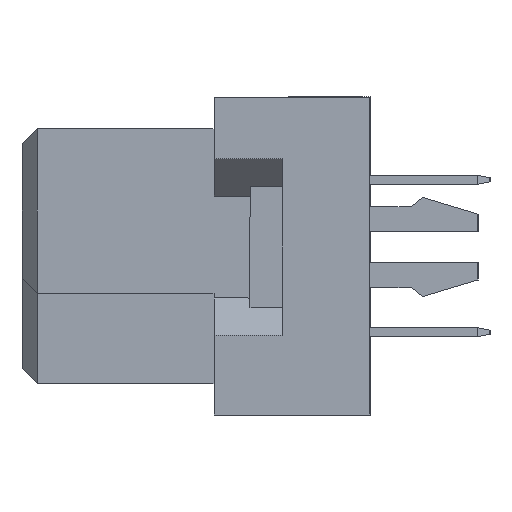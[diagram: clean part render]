
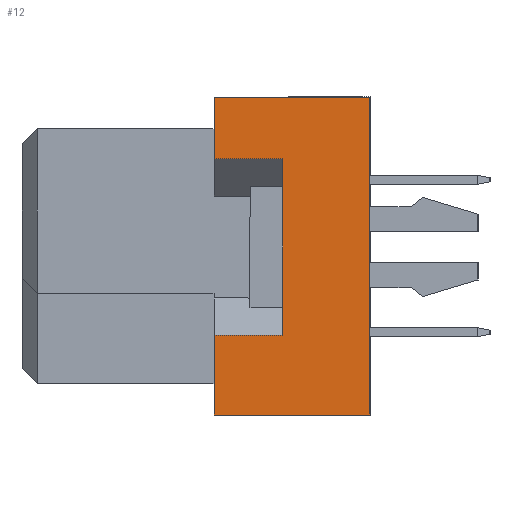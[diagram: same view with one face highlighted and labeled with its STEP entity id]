
A CAD part, left-side view. The second image highlights one B-rep face of the part: STEP entity #12.
In plain terms, the highlighted planar face has unit normal (-1, 0, 0).
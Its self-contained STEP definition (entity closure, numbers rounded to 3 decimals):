
#12 = ADVANCED_FACE ( 'NONE', ( #2517 ), #5895, .T. ) ;
#222 = EDGE_CURVE ( 'NONE', #2448, #16559, #4938, .T. ) ;
#498 = DIRECTION ( 'NONE',  ( 0., 0., 1. ) ) ;
#691 = EDGE_CURVE ( 'NONE', #2448, #20580, #8962, .T. ) ;
#697 = DIRECTION ( 'NONE',  ( 0., 0., 1. ) ) ;
#1095 = CARTESIAN_POINT ( 'NONE',  ( -27.5, -8.7, 3.25 ) ) ;
#1193 = DIRECTION ( 'NONE',  ( 0., 1., 0. ) ) ;
#1994 = VERTEX_POINT ( 'NONE', #15630 ) ;
#2054 = VECTOR ( 'NONE', #9783, 1000. ) ;
#2367 = VECTOR ( 'NONE', #697, 1000. ) ;
#2448 = VERTEX_POINT ( 'NONE', #15815 ) ;
#2517 = FACE_OUTER_BOUND ( 'NONE', #18444, .T. ) ;
#2866 = VERTEX_POINT ( 'NONE', #7513 ) ;
#3087 = VECTOR ( 'NONE', #9484, 1000. ) ;
#3811 = VECTOR ( 'NONE', #498, 1000. ) ;
#3842 = CARTESIAN_POINT ( 'NONE',  ( -27.5, -11.6, -5.3 ) ) ;
#3934 = ORIENTED_EDGE ( 'NONE', *, *, #18700, .T. ) ;
#4005 = AXIS2_PLACEMENT_3D ( 'NONE', #10819, #9157, #9797 ) ;
#4315 = ORIENTED_EDGE ( 'NONE', *, *, #8371, .F. ) ;
#4316 = VECTOR ( 'NONE', #1193, 1000. ) ;
#4778 = LINE ( 'NONE', #1095, #4316 ) ;
#4833 = CARTESIAN_POINT ( 'NONE',  ( -27.5, -11.6, 5.3 ) ) ;
#4938 = LINE ( 'NONE', #4833, #7492 ) ;
#4966 = CARTESIAN_POINT ( 'NONE',  ( -27.5, -11.6, 5.3 ) ) ;
#5068 = CARTESIAN_POINT ( 'NONE',  ( -27.5, -8.7, -2.65 ) ) ;
#5236 = CARTESIAN_POINT ( 'NONE',  ( -27.5, -11.6, 5.3 ) ) ;
#5796 = DIRECTION ( 'NONE',  ( 0., 1., 0. ) ) ;
#5895 = PLANE ( 'NONE',  #4005 ) ;
#6091 = VERTEX_POINT ( 'NONE', #11213 ) ;
#6583 = DIRECTION ( 'NONE',  ( 0., 0., 1. ) ) ;
#6626 = ORIENTED_EDGE ( 'NONE', *, *, #222, .T. ) ;
#7226 = EDGE_CURVE ( 'NONE', #2866, #18574, #7423, .T. ) ;
#7423 = LINE ( 'NONE', #11024, #3087 ) ;
#7492 = VECTOR ( 'NONE', #6583, 1000. ) ;
#7513 = CARTESIAN_POINT ( 'NONE',  ( -27.5, -8.7, -2.65 ) ) ;
#7664 = CARTESIAN_POINT ( 'NONE',  ( -27.5, -6.4, -5.3 ) ) ;
#7937 = ORIENTED_EDGE ( 'NONE', *, *, #13612, .F. ) ;
#8371 = EDGE_CURVE ( 'NONE', #2866, #1994, #13483, .T. ) ;
#8962 = LINE ( 'NONE', #3842, #12075 ) ;
#9157 = DIRECTION ( 'NONE',  ( -1., 0., 0. ) ) ;
#9484 = DIRECTION ( 'NONE',  ( 0., 1., 0. ) ) ;
#9783 = DIRECTION ( 'NONE',  ( 0., 1., 0. ) ) ;
#9797 = DIRECTION ( 'NONE',  ( 0., 0., 1. ) ) ;
#9897 = VERTEX_POINT ( 'NONE', #17917 ) ;
#10819 = CARTESIAN_POINT ( 'NONE',  ( -27.5, -11.6, 5.3 ) ) ;
#11024 = CARTESIAN_POINT ( 'NONE',  ( -27.5, -8.7, -2.65 ) ) ;
#11100 = CARTESIAN_POINT ( 'NONE',  ( -27.5, -6.4, -2.65 ) ) ;
#11213 = CARTESIAN_POINT ( 'NONE',  ( -27.5, -6.4, 5.3 ) ) ;
#12075 = VECTOR ( 'NONE', #5796, 1000. ) ;
#12771 = EDGE_CURVE ( 'NONE', #1994, #9897, #4778, .T. ) ;
#13483 = LINE ( 'NONE', #5068, #3811 ) ;
#13612 = EDGE_CURVE ( 'NONE', #20580, #18574, #20847, .T. ) ;
#13688 = ORIENTED_EDGE ( 'NONE', *, *, #7226, .T. ) ;
#14242 = DIRECTION ( 'NONE',  ( 0., 0., 1. ) ) ;
#14506 = ORIENTED_EDGE ( 'NONE', *, *, #691, .F. ) ;
#15394 = ORIENTED_EDGE ( 'NONE', *, *, #12771, .F. ) ;
#15630 = CARTESIAN_POINT ( 'NONE',  ( -27.5, -8.7, 3.25 ) ) ;
#15815 = CARTESIAN_POINT ( 'NONE',  ( -27.5, -11.6, -5.3 ) ) ;
#16559 = VERTEX_POINT ( 'NONE', #5236 ) ;
#17012 = CARTESIAN_POINT ( 'NONE',  ( -27.5, -6.4, -5.3 ) ) ;
#17616 = ORIENTED_EDGE ( 'NONE', *, *, #19419, .F. ) ;
#17822 = CARTESIAN_POINT ( 'NONE',  ( -27.5, -6.4, -5.3 ) ) ;
#17917 = CARTESIAN_POINT ( 'NONE',  ( -27.5, -6.4, 3.25 ) ) ;
#18263 = LINE ( 'NONE', #4966, #2054 ) ;
#18444 = EDGE_LOOP ( 'NONE', ( #13688, #7937, #14506, #6626, #3934, #17616, #15394, #4315 ) ) ;
#18574 = VERTEX_POINT ( 'NONE', #11100 ) ;
#18700 = EDGE_CURVE ( 'NONE', #16559, #6091, #18263, .T. ) ;
#18973 = LINE ( 'NONE', #7664, #2367 ) ;
#19419 = EDGE_CURVE ( 'NONE', #9897, #6091, #18973, .T. ) ;
#20580 = VERTEX_POINT ( 'NONE', #17012 ) ;
#20589 = VECTOR ( 'NONE', #14242, 1000. ) ;
#20847 = LINE ( 'NONE', #17822, #20589 ) ;
